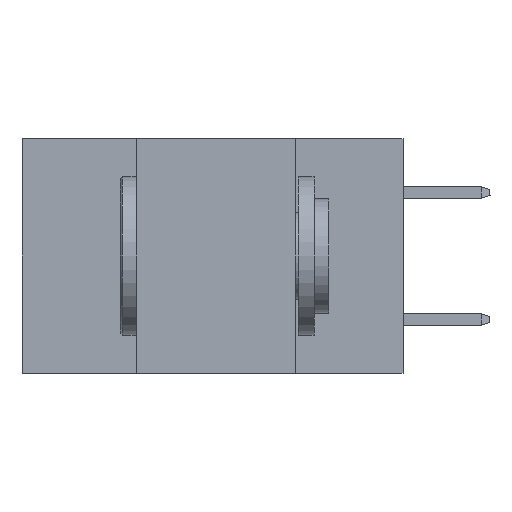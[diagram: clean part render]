
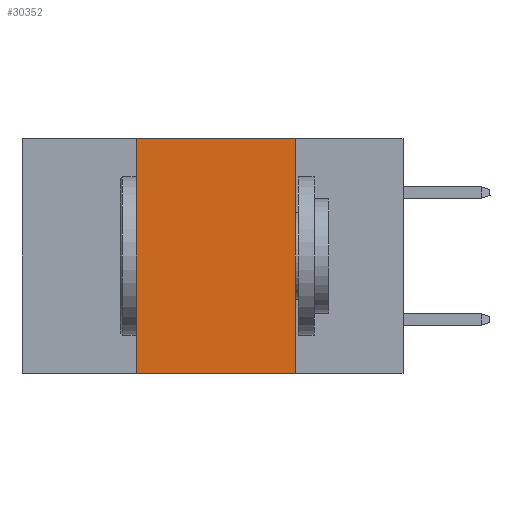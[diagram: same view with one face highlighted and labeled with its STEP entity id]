
A CAD part, left-side view. The second image highlights one B-rep face of the part: STEP entity #30352.
In plain terms, the highlighted planar face has unit normal (-1, 0, 0).
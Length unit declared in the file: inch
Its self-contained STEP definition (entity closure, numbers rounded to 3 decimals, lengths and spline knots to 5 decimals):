
#2896 = LINE ( 'NONE', #31275, #27847 ) ;
#3050 = LINE ( 'NONE', #16447, #3392 ) ;
#3392 = VECTOR ( 'NONE', #45234, 39.37008 ) ;
#4790 = EDGE_LOOP ( 'NONE', ( #37977, #31906, #37853, #9298 ) ) ;
#5673 = FACE_OUTER_BOUND ( 'NONE', #4790, .T. ) ;
#6851 = EDGE_CURVE ( 'NONE', #29158, #35360, #2896, .T. ) ;
#8331 = VECTOR ( 'NONE', #17444, 39.37008 ) ;
#9298 = ORIENTED_EDGE ( 'NONE', *, *, #37764, .T. ) ;
#11365 = LINE ( 'NONE', #15267, #30424 ) ;
#13310 = CARTESIAN_POINT ( 'NONE',  ( 0., 0.6, 0. ) ) ;
#15267 = CARTESIAN_POINT ( 'NONE',  ( 0., 0.17, 0. ) ) ;
#16447 = CARTESIAN_POINT ( 'NONE',  ( 0., 0.42, 0. ) ) ;
#16988 = DIRECTION ( 'NONE',  ( 0., -1., 0. ) ) ;
#17444 = DIRECTION ( 'NONE',  ( 0., -1., 0. ) ) ;
#18522 = LINE ( 'NONE', #24366, #8331 ) ;
#19780 = DIRECTION ( 'NONE',  ( 0., 0., -1. ) ) ;
#20380 = CARTESIAN_POINT ( 'NONE',  ( 0., 0.17, -0.37 ) ) ;
#21658 = EDGE_CURVE ( 'NONE', #35360, #35117, #11365, .T. ) ;
#22438 = DIRECTION ( 'NONE',  ( 0., 0., -1. ) ) ;
#23927 = PLANE ( 'NONE',  #25637 ) ;
#24366 = CARTESIAN_POINT ( 'NONE',  ( 0., 0.6, -0.37 ) ) ;
#25197 = CARTESIAN_POINT ( 'NONE',  ( 0., 0.17, 0. ) ) ;
#25327 = VERTEX_POINT ( 'NONE', #25403 ) ;
#25403 = CARTESIAN_POINT ( 'NONE',  ( 0., 0.42, -0.37 ) ) ;
#25637 = AXIS2_PLACEMENT_3D ( 'NONE', #13310, #30159, #19780 ) ;
#27847 = VECTOR ( 'NONE', #16988, 39.37008 ) ;
#28380 = EDGE_CURVE ( 'NONE', #25327, #29158, #3050, .T. ) ;
#29158 = VERTEX_POINT ( 'NONE', #40933 ) ;
#30159 = DIRECTION ( 'NONE',  ( 1., 0., 0. ) ) ;
#30352 = ADVANCED_FACE ( 'NONE', ( #5673 ), #23927, .F. ) ;
#30424 = VECTOR ( 'NONE', #22438, 39.37008 ) ;
#31275 = CARTESIAN_POINT ( 'NONE',  ( 0., 0.6, 0. ) ) ;
#31906 = ORIENTED_EDGE ( 'NONE', *, *, #6851, .F. ) ;
#35117 = VERTEX_POINT ( 'NONE', #20380 ) ;
#35360 = VERTEX_POINT ( 'NONE', #25197 ) ;
#37764 = EDGE_CURVE ( 'NONE', #25327, #35117, #18522, .T. ) ;
#37853 = ORIENTED_EDGE ( 'NONE', *, *, #28380, .F. ) ;
#37977 = ORIENTED_EDGE ( 'NONE', *, *, #21658, .F. ) ;
#40933 = CARTESIAN_POINT ( 'NONE',  ( 0., 0.42, 0. ) ) ;
#45234 = DIRECTION ( 'NONE',  ( 0., 0., 1. ) ) ;
